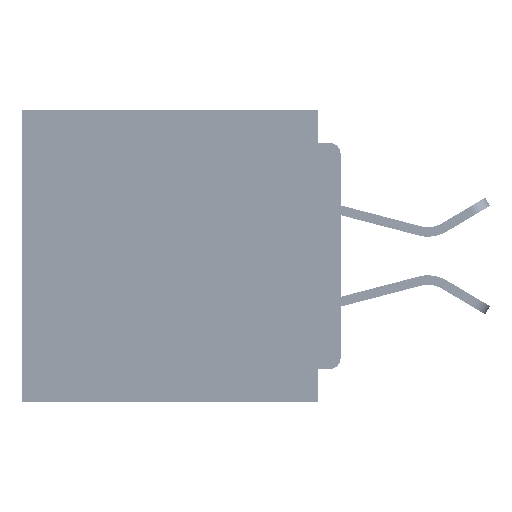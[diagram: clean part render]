
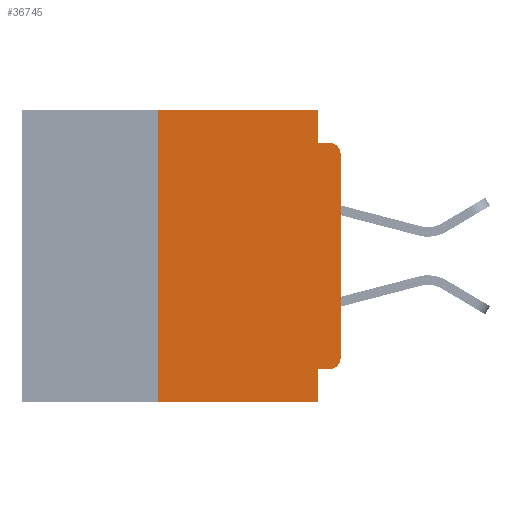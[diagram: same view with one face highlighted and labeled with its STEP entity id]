
A CAD part, left-side view. The second image highlights one B-rep face of the part: STEP entity #36745.
In plain terms, the highlighted planar face has unit normal (-1, 0, 0).
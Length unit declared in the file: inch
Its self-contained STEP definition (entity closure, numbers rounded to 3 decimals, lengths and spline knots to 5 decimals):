
#186 = AXIS2_PLACEMENT_3D ( 'NONE', #8015, #40419, #12621 ) ;
#902 = CARTESIAN_POINT ( 'NONE',  ( 0., 0.015, -0.06 ) ) ;
#1467 = VERTEX_POINT ( 'NONE', #53265 ) ;
#3219 = AXIS2_PLACEMENT_3D ( 'NONE', #902, #33408, #5642 ) ;
#3357 = ORIENTED_EDGE ( 'NONE', *, *, #22789, .T. ) ;
#3971 = LINE ( 'NONE', #8141, #53308 ) ;
#5079 = CARTESIAN_POINT ( 'NONE',  ( 0., 0.437, 0. ) ) ;
#5642 = DIRECTION ( 'NONE',  ( 0., 0., -1. ) ) ;
#5904 = VERTEX_POINT ( 'NONE', #34862 ) ;
#6102 = DIRECTION ( 'NONE',  ( 0., 0., -1. ) ) ;
#6446 = CARTESIAN_POINT ( 'NONE',  ( 0., 0.437, -0.4 ) ) ;
#6474 = LINE ( 'NONE', #59109, #25257 ) ;
#6715 = EDGE_LOOP ( 'NONE', ( #36072, #3357, #41633, #43793, #16454, #49541, #36520, #59380, #38951, #25905 ) ) ;
#6815 = VECTOR ( 'NONE', #45047, 39.37008 ) ;
#8015 = CARTESIAN_POINT ( 'NONE',  ( 0., 0.015, -0.34 ) ) ;
#8134 = DIRECTION ( 'NONE',  ( 0., 1., 0. ) ) ;
#8141 = CARTESIAN_POINT ( 'NONE',  ( 0., 0.25, -0.4 ) ) ;
#8251 = LINE ( 'NONE', #54359, #6815 ) ;
#8315 = VERTEX_POINT ( 'NONE', #53865 ) ;
#9208 = LINE ( 'NONE', #6446, #55581 ) ;
#9748 = DIRECTION ( 'NONE',  ( 1., 0., 0. ) ) ;
#11535 = LINE ( 'NONE', #34267, #12989 ) ;
#12375 = DIRECTION ( 'NONE',  ( 0., -1., 0. ) ) ;
#12621 = DIRECTION ( 'NONE',  ( 0., 0., -1. ) ) ;
#12989 = VECTOR ( 'NONE', #25118, 39.37008 ) ;
#14178 = PLANE ( 'NONE',  #21455 ) ;
#15618 = CARTESIAN_POINT ( 'NONE',  ( 0., 0.015, -0.045 ) ) ;
#16031 = VECTOR ( 'NONE', #12375, 39.37008 ) ;
#16454 = ORIENTED_EDGE ( 'NONE', *, *, #36497, .F. ) ;
#16543 = CARTESIAN_POINT ( 'NONE',  ( 0., 0.031, -0.045 ) ) ;
#18181 = FACE_OUTER_BOUND ( 'NONE', #6715, .T. ) ;
#18609 = EDGE_CURVE ( 'NONE', #40288, #52865, #6474, .T. ) ;
#19111 = VERTEX_POINT ( 'NONE', #16543 ) ;
#19466 = VECTOR ( 'NONE', #6102, 39.37008 ) ;
#20397 = EDGE_CURVE ( 'NONE', #1467, #5904, #3971, .T. ) ;
#21455 = AXIS2_PLACEMENT_3D ( 'NONE', #5079, #9748, #42173 ) ;
#21852 = EDGE_CURVE ( 'NONE', #8315, #28178, #8251, .T. ) ;
#22097 = CIRCLE ( 'NONE', #186, 0.015 ) ;
#22789 = EDGE_CURVE ( 'NONE', #28178, #39150, #25485, .T. ) ;
#24126 = EDGE_CURVE ( 'NONE', #35671, #19111, #11535, .T. ) ;
#25118 = DIRECTION ( 'NONE',  ( 0., 0., -1. ) ) ;
#25257 = VECTOR ( 'NONE', #8134, 39.37008 ) ;
#25485 = CIRCLE ( 'NONE', #3219, 0.015 ) ;
#25566 = EDGE_CURVE ( 'NONE', #19111, #39150, #27302, .T. ) ;
#25905 = ORIENTED_EDGE ( 'NONE', *, *, #40547, .T. ) ;
#26878 = CARTESIAN_POINT ( 'NONE',  ( 0., 0.031, 0. ) ) ;
#27302 = LINE ( 'NONE', #58576, #54872 ) ;
#28178 = VERTEX_POINT ( 'NONE', #44681 ) ;
#28532 = CARTESIAN_POINT ( 'NONE',  ( 0., 0.031, -0.355 ) ) ;
#29166 = CARTESIAN_POINT ( 'NONE',  ( 0., 0.031, -0.4 ) ) ;
#29815 = LINE ( 'NONE', #58752, #16031 ) ;
#30947 = CARTESIAN_POINT ( 'NONE',  ( 0., 0.031, -0.4 ) ) ;
#33408 = DIRECTION ( 'NONE',  ( -1., 0., 0. ) ) ;
#33765 = CARTESIAN_POINT ( 'NONE',  ( 0., 0.015, -0.355 ) ) ;
#34267 = CARTESIAN_POINT ( 'NONE',  ( 0., 0.031, 0. ) ) ;
#34862 = CARTESIAN_POINT ( 'NONE',  ( 0., 0.25, 0. ) ) ;
#35548 = DIRECTION ( 'NONE',  ( 0., -1., 0. ) ) ;
#35671 = VERTEX_POINT ( 'NONE', #26878 ) ;
#36072 = ORIENTED_EDGE ( 'NONE', *, *, #21852, .T. ) ;
#36497 = EDGE_CURVE ( 'NONE', #5904, #35671, #29815, .T. ) ;
#36520 = ORIENTED_EDGE ( 'NONE', *, *, #45470, .T. ) ;
#36745 = ADVANCED_FACE ( 'NONE', ( #18181 ), #14178, .F. ) ;
#38951 = ORIENTED_EDGE ( 'NONE', *, *, #18609, .F. ) ;
#39150 = VERTEX_POINT ( 'NONE', #15618 ) ;
#39251 = DIRECTION ( 'NONE',  ( 0., -1., 0. ) ) ;
#40288 = VERTEX_POINT ( 'NONE', #33765 ) ;
#40419 = DIRECTION ( 'NONE',  ( -1., 0., 0. ) ) ;
#40547 = EDGE_CURVE ( 'NONE', #40288, #8315, #22097, .T. ) ;
#41633 = ORIENTED_EDGE ( 'NONE', *, *, #25566, .F. ) ;
#41816 = VERTEX_POINT ( 'NONE', #30947 ) ;
#42173 = DIRECTION ( 'NONE',  ( 0., 0., -1. ) ) ;
#43793 = ORIENTED_EDGE ( 'NONE', *, *, #24126, .F. ) ;
#44681 = CARTESIAN_POINT ( 'NONE',  ( 0., 0., -0.06 ) ) ;
#45047 = DIRECTION ( 'NONE',  ( 0., 0., 1. ) ) ;
#45195 = DIRECTION ( 'NONE',  ( 0., 0., 1. ) ) ;
#45470 = EDGE_CURVE ( 'NONE', #1467, #41816, #9208, .T. ) ;
#49541 = ORIENTED_EDGE ( 'NONE', *, *, #20397, .F. ) ;
#51030 = EDGE_CURVE ( 'NONE', #52865, #41816, #59283, .T. ) ;
#52865 = VERTEX_POINT ( 'NONE', #28532 ) ;
#53265 = CARTESIAN_POINT ( 'NONE',  ( 0., 0.25, -0.4 ) ) ;
#53308 = VECTOR ( 'NONE', #45195, 39.37008 ) ;
#53865 = CARTESIAN_POINT ( 'NONE',  ( 0., 0., -0.34 ) ) ;
#54359 = CARTESIAN_POINT ( 'NONE',  ( 0., 0., 0. ) ) ;
#54872 = VECTOR ( 'NONE', #35548, 39.37008 ) ;
#55581 = VECTOR ( 'NONE', #39251, 39.37008 ) ;
#58576 = CARTESIAN_POINT ( 'NONE',  ( 0., 0., -0.045 ) ) ;
#58752 = CARTESIAN_POINT ( 'NONE',  ( 0., 0.437, 0. ) ) ;
#59109 = CARTESIAN_POINT ( 'NONE',  ( 0., 0., -0.355 ) ) ;
#59283 = LINE ( 'NONE', #29166, #19466 ) ;
#59380 = ORIENTED_EDGE ( 'NONE', *, *, #51030, .F. ) ;
